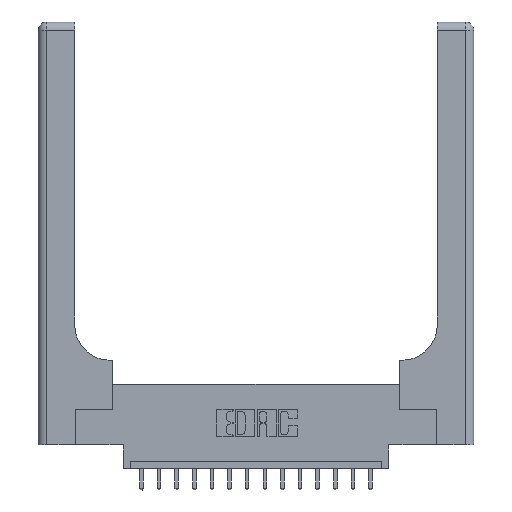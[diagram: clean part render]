
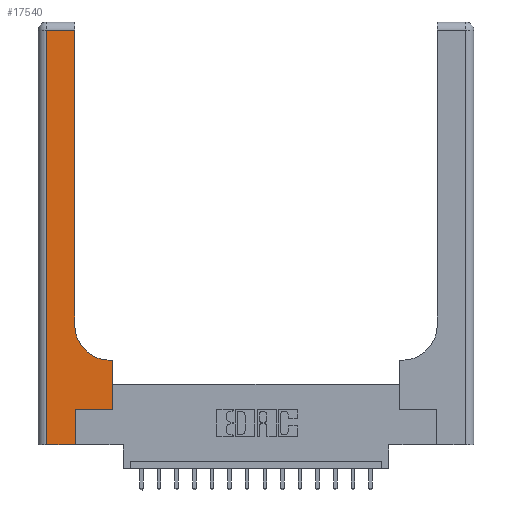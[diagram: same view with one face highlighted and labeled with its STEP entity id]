
A CAD part, top view. The second image highlights one B-rep face of the part: STEP entity #17540.
In plain terms, the highlighted planar face has unit normal (0, 0, 1).
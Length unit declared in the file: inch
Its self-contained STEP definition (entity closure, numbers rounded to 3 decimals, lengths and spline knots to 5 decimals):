
#204 = LINE ( 'NONE', #8118, #13936 ) ;
#625 = CARTESIAN_POINT ( 'NONE',  ( 0.06, 0., 0.37 ) ) ;
#1221 = VERTEX_POINT ( 'NONE', #3129 ) ;
#1374 = VERTEX_POINT ( 'NONE', #8960 ) ;
#2019 = CARTESIAN_POINT ( 'NONE',  ( 0., 0., 0.37 ) ) ;
#2353 = EDGE_CURVE ( 'NONE', #13995, #11406, #4407, .T. ) ;
#2725 = CARTESIAN_POINT ( 'NONE',  ( 0., 3., 0.37 ) ) ;
#2847 = VECTOR ( 'NONE', #8180, 39.37008 ) ;
#3035 = PLANE ( 'NONE',  #13579 ) ;
#3129 = CARTESIAN_POINT ( 'NONE',  ( 0.26, 0.85, 0.37 ) ) ;
#3160 = EDGE_LOOP ( 'NONE', ( #4722, #4534, #5849, #12692, #11172, #15912, #12373, #11912, #5977 ) ) ;
#3773 = CIRCLE ( 'NONE', #15659, 0.25 ) ;
#4136 = DIRECTION ( 'NONE',  ( 0., 1., 0. ) ) ;
#4407 = LINE ( 'NONE', #8846, #17538 ) ;
#4413 = CARTESIAN_POINT ( 'NONE',  ( 0.528, 0.6, 0.37 ) ) ;
#4534 = ORIENTED_EDGE ( 'NONE', *, *, #2353, .T. ) ;
#4585 = CARTESIAN_POINT ( 'NONE',  ( 0.265, 0., 0.37 ) ) ;
#4722 = ORIENTED_EDGE ( 'NONE', *, *, #6090, .T. ) ;
#4955 = VERTEX_POINT ( 'NONE', #17785 ) ;
#5514 = DIRECTION ( 'NONE',  ( 0., 0., -1. ) ) ;
#5777 = CARTESIAN_POINT ( 'NONE',  ( 0.26, 0.6, 0.37 ) ) ;
#5849 = ORIENTED_EDGE ( 'NONE', *, *, #6793, .T. ) ;
#5977 = ORIENTED_EDGE ( 'NONE', *, *, #15434, .T. ) ;
#6090 = EDGE_CURVE ( 'NONE', #1221, #13995, #204, .T. ) ;
#6390 = VECTOR ( 'NONE', #14212, 39.37008 ) ;
#6573 = CARTESIAN_POINT ( 'NONE',  ( 0.51, 0.6, 0.37 ) ) ;
#6643 = CARTESIAN_POINT ( 'NONE',  ( 0.265, 0.25, 0.37 ) ) ;
#6793 = EDGE_CURVE ( 'NONE', #11406, #13993, #8143, .T. ) ;
#6900 = VERTEX_POINT ( 'NONE', #6643 ) ;
#6926 = VERTEX_POINT ( 'NONE', #6573 ) ;
#7445 = VECTOR ( 'NONE', #12542, 39.37008 ) ;
#7539 = DIRECTION ( 'NONE',  ( 0., -1., 0. ) ) ;
#7839 = EDGE_CURVE ( 'NONE', #6900, #1374, #17679, .T. ) ;
#8118 = CARTESIAN_POINT ( 'NONE',  ( 0.26, 3., 0.37 ) ) ;
#8143 = LINE ( 'NONE', #17342, #10947 ) ;
#8177 = DIRECTION ( 'NONE',  ( 0., 1., 0. ) ) ;
#8180 = DIRECTION ( 'NONE',  ( 1., 0., 0. ) ) ;
#8846 = CARTESIAN_POINT ( 'NONE',  ( 0., 2.94, 0.37 ) ) ;
#8960 = CARTESIAN_POINT ( 'NONE',  ( 0.528, 0.25, 0.37 ) ) ;
#9170 = CARTESIAN_POINT ( 'NONE',  ( 0.265, 0.25, 0.37 ) ) ;
#9859 = VECTOR ( 'NONE', #4136, 39.37008 ) ;
#10360 = CARTESIAN_POINT ( 'NONE',  ( 0.06, 2.94, 0.37 ) ) ;
#10947 = VECTOR ( 'NONE', #7539, 39.37008 ) ;
#11125 = LINE ( 'NONE', #5777, #7445 ) ;
#11172 = ORIENTED_EDGE ( 'NONE', *, *, #11403, .T. ) ;
#11393 = LINE ( 'NONE', #12205, #9859 ) ;
#11403 = EDGE_CURVE ( 'NONE', #4955, #6900, #15713, .T. ) ;
#11406 = VERTEX_POINT ( 'NONE', #10360 ) ;
#11894 = VECTOR ( 'NONE', #15844, 39.37008 ) ;
#11912 = ORIENTED_EDGE ( 'NONE', *, *, #15532, .T. ) ;
#12205 = CARTESIAN_POINT ( 'NONE',  ( 0.528, 0.25, 0.37 ) ) ;
#12373 = ORIENTED_EDGE ( 'NONE', *, *, #12728, .T. ) ;
#12488 = FACE_OUTER_BOUND ( 'NONE', #3160, .T. ) ;
#12542 = DIRECTION ( 'NONE',  ( -1., 0., 0. ) ) ;
#12692 = ORIENTED_EDGE ( 'NONE', *, *, #16085, .T. ) ;
#12728 = EDGE_CURVE ( 'NONE', #1374, #16121, #11393, .T. ) ;
#12903 = CARTESIAN_POINT ( 'NONE',  ( 0.26, 2.94, 0.37 ) ) ;
#12990 = DIRECTION ( 'NONE',  ( -1., 0., 0. ) ) ;
#13579 = AXIS2_PLACEMENT_3D ( 'NONE', #2725, #17680, #16378 ) ;
#13631 = CARTESIAN_POINT ( 'NONE',  ( 0.51, 0.85, 0.37 ) ) ;
#13936 = VECTOR ( 'NONE', #8177, 39.37008 ) ;
#13993 = VERTEX_POINT ( 'NONE', #625 ) ;
#13995 = VERTEX_POINT ( 'NONE', #12903 ) ;
#14212 = DIRECTION ( 'NONE',  ( 0., 1., 0. ) ) ;
#15434 = EDGE_CURVE ( 'NONE', #6926, #1221, #3773, .T. ) ;
#15532 = EDGE_CURVE ( 'NONE', #16121, #6926, #11125, .T. ) ;
#15659 = AXIS2_PLACEMENT_3D ( 'NONE', #13631, #5514, #16820 ) ;
#15713 = LINE ( 'NONE', #4585, #6390 ) ;
#15844 = DIRECTION ( 'NONE',  ( 1., 0., 0. ) ) ;
#15912 = ORIENTED_EDGE ( 'NONE', *, *, #7839, .T. ) ;
#16085 = EDGE_CURVE ( 'NONE', #13993, #4955, #16652, .T. ) ;
#16121 = VERTEX_POINT ( 'NONE', #4413 ) ;
#16378 = DIRECTION ( 'NONE',  ( -1., 0., 0. ) ) ;
#16652 = LINE ( 'NONE', #2019, #11894 ) ;
#16820 = DIRECTION ( 'NONE',  ( 1., 0., 0. ) ) ;
#17342 = CARTESIAN_POINT ( 'NONE',  ( 0.06, 3., 0.37 ) ) ;
#17538 = VECTOR ( 'NONE', #12990, 39.37008 ) ;
#17540 = ADVANCED_FACE ( 'NONE', ( #12488 ), #3035, .F. ) ;
#17679 = LINE ( 'NONE', #9170, #2847 ) ;
#17680 = DIRECTION ( 'NONE',  ( 0., 0., -1. ) ) ;
#17785 = CARTESIAN_POINT ( 'NONE',  ( 0.265, 0., 0.37 ) ) ;
